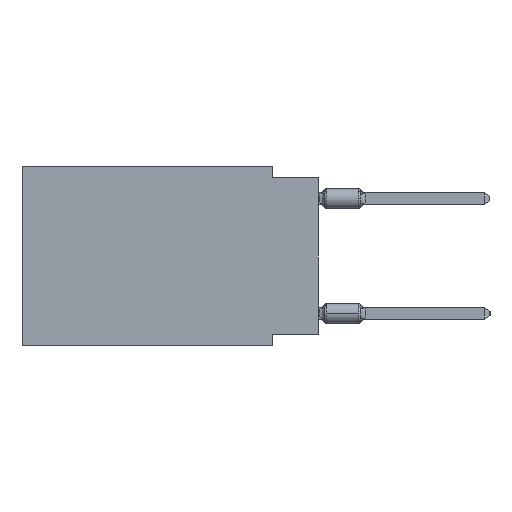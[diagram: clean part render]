
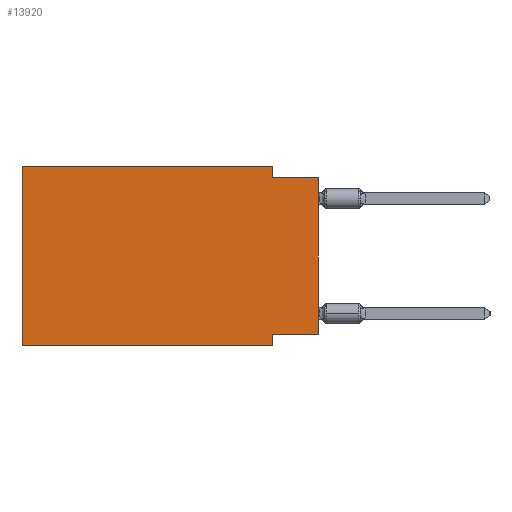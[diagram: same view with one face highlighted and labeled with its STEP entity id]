
A CAD part, left-side view. The second image highlights one B-rep face of the part: STEP entity #13920.
In plain terms, the highlighted planar face has unit normal (-1, 0, 0).
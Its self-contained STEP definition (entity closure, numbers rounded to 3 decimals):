
#926 = EDGE_CURVE ( 'NONE', #17552, #12842, #27835, .T. ) ;
#2417 = LINE ( 'NONE', #25408, #5070 ) ;
#2421 = DIRECTION ( 'NONE',  ( 0., 0., 1. ) ) ;
#3348 = AXIS2_PLACEMENT_3D ( 'NONE', #37544, #11072, #14166 ) ;
#3723 = CARTESIAN_POINT ( 'NONE',  ( 0., 2.54, 0. ) ) ;
#3798 = VERTEX_POINT ( 'NONE', #5365 ) ;
#5070 = VECTOR ( 'NONE', #13610, 1000. ) ;
#5159 = VECTOR ( 'NONE', #28958, 1000. ) ;
#5365 = CARTESIAN_POINT ( 'NONE',  ( 0., 2.54, -0.635 ) ) ;
#6780 = DIRECTION ( 'NONE',  ( 0., 1., 0. ) ) ;
#7075 = ORIENTED_EDGE ( 'NONE', *, *, #30914, .T. ) ;
#8021 = VERTEX_POINT ( 'NONE', #15417 ) ;
#9002 = LINE ( 'NONE', #32592, #28908 ) ;
#9728 = VECTOR ( 'NONE', #30921, 1000. ) ;
#9936 = ORIENTED_EDGE ( 'NONE', *, *, #12209, .T. ) ;
#10101 = EDGE_CURVE ( 'NONE', #12842, #3798, #2417, .T. ) ;
#10428 = CARTESIAN_POINT ( 'NONE',  ( 0., 0., -9.271 ) ) ;
#10719 = VECTOR ( 'NONE', #28462, 1000. ) ;
#11066 = CARTESIAN_POINT ( 'NONE',  ( 0., 16.383, 0. ) ) ;
#11072 = DIRECTION ( 'NONE',  ( 1., 0., 0. ) ) ;
#11287 = VERTEX_POINT ( 'NONE', #16391 ) ;
#11366 = CARTESIAN_POINT ( 'NONE',  ( 0., 2.54, -9.906 ) ) ;
#12209 = EDGE_CURVE ( 'NONE', #27080, #23127, #22545, .T. ) ;
#12842 = VERTEX_POINT ( 'NONE', #3723 ) ;
#13525 = CARTESIAN_POINT ( 'NONE',  ( 0., 16.383, 0. ) ) ;
#13610 = DIRECTION ( 'NONE',  ( 0., 0., -1. ) ) ;
#13858 = EDGE_CURVE ( 'NONE', #3798, #23127, #37155, .T. ) ;
#13920 = ADVANCED_FACE ( 'NONE', ( #28862 ), #25767, .F. ) ;
#14166 = DIRECTION ( 'NONE',  ( 0., 0., -1. ) ) ;
#15417 = CARTESIAN_POINT ( 'NONE',  ( 0., 2.54, -9.271 ) ) ;
#16391 = CARTESIAN_POINT ( 'NONE',  ( 0., 2.54, -9.906 ) ) ;
#16535 = CARTESIAN_POINT ( 'NONE',  ( 0., 16.383, -9.906 ) ) ;
#17412 = EDGE_LOOP ( 'NONE', ( #9936, #26437, #25289, #37055, #36283, #7075, #28767, #24122 ) ) ;
#17552 = VERTEX_POINT ( 'NONE', #11066 ) ;
#18035 = VECTOR ( 'NONE', #2421, 1000. ) ;
#18292 = EDGE_CURVE ( 'NONE', #8021, #11287, #19870, .T. ) ;
#19324 = LINE ( 'NONE', #10428, #19728 ) ;
#19728 = VECTOR ( 'NONE', #6780, 1000. ) ;
#19870 = LINE ( 'NONE', #11366, #5159 ) ;
#20418 = DIRECTION ( 'NONE',  ( 0., -1., 0. ) ) ;
#21066 = VERTEX_POINT ( 'NONE', #16535 ) ;
#21555 = EDGE_CURVE ( 'NONE', #21066, #17552, #37002, .T. ) ;
#22545 = LINE ( 'NONE', #31044, #34087 ) ;
#23127 = VERTEX_POINT ( 'NONE', #37470 ) ;
#23811 = CARTESIAN_POINT ( 'NONE',  ( 0., 0., -9.271 ) ) ;
#24122 = ORIENTED_EDGE ( 'NONE', *, *, #32801, .F. ) ;
#25289 = ORIENTED_EDGE ( 'NONE', *, *, #10101, .F. ) ;
#25408 = CARTESIAN_POINT ( 'NONE',  ( 0., 2.54, 0. ) ) ;
#25580 = CARTESIAN_POINT ( 'NONE',  ( 0., 0., -0.635 ) ) ;
#25767 = PLANE ( 'NONE',  #3348 ) ;
#25807 = CARTESIAN_POINT ( 'NONE',  ( 0., 16.383, 0. ) ) ;
#26437 = ORIENTED_EDGE ( 'NONE', *, *, #13858, .F. ) ;
#27080 = VERTEX_POINT ( 'NONE', #23811 ) ;
#27835 = LINE ( 'NONE', #13525, #9728 ) ;
#28462 = DIRECTION ( 'NONE',  ( 0., -1., 0. ) ) ;
#28767 = ORIENTED_EDGE ( 'NONE', *, *, #18292, .F. ) ;
#28862 = FACE_OUTER_BOUND ( 'NONE', #17412, .T. ) ;
#28908 = VECTOR ( 'NONE', #20418, 1000. ) ;
#28958 = DIRECTION ( 'NONE',  ( 0., 0., -1. ) ) ;
#30914 = EDGE_CURVE ( 'NONE', #21066, #11287, #9002, .T. ) ;
#30921 = DIRECTION ( 'NONE',  ( 0., -1., 0. ) ) ;
#31044 = CARTESIAN_POINT ( 'NONE',  ( 0., 0., 0. ) ) ;
#32592 = CARTESIAN_POINT ( 'NONE',  ( 0., 16.383, -9.906 ) ) ;
#32801 = EDGE_CURVE ( 'NONE', #27080, #8021, #19324, .T. ) ;
#34087 = VECTOR ( 'NONE', #34331, 1000. ) ;
#34331 = DIRECTION ( 'NONE',  ( 0., 0., 1. ) ) ;
#36283 = ORIENTED_EDGE ( 'NONE', *, *, #21555, .F. ) ;
#37002 = LINE ( 'NONE', #25807, #18035 ) ;
#37055 = ORIENTED_EDGE ( 'NONE', *, *, #926, .F. ) ;
#37155 = LINE ( 'NONE', #25580, #10719 ) ;
#37470 = CARTESIAN_POINT ( 'NONE',  ( 0., 0., -0.635 ) ) ;
#37544 = CARTESIAN_POINT ( 'NONE',  ( 0., 16.383, 0. ) ) ;
